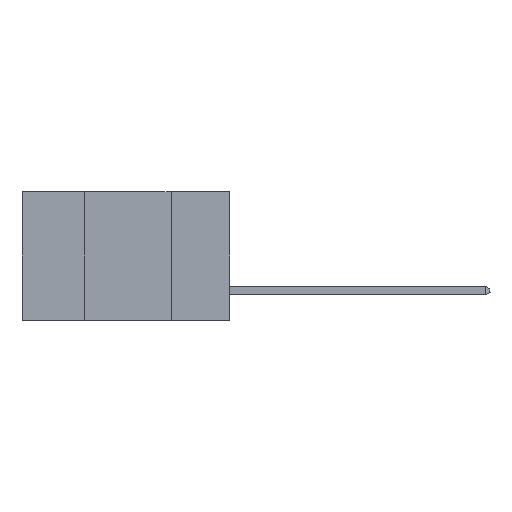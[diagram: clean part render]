
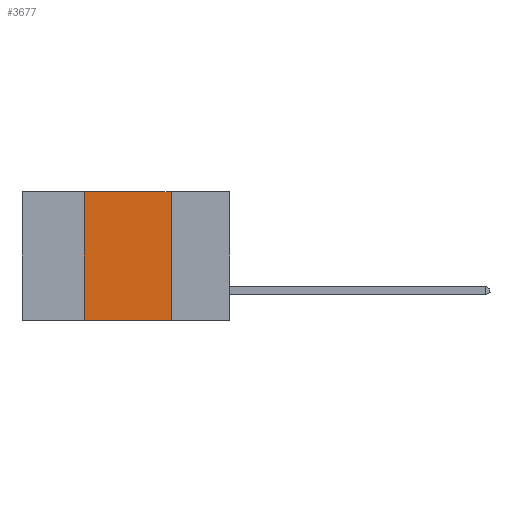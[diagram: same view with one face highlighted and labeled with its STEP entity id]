
A CAD part, left-side view. The second image highlights one B-rep face of the part: STEP entity #3677.
In plain terms, the highlighted planar face has unit normal (-1, 0, 0).
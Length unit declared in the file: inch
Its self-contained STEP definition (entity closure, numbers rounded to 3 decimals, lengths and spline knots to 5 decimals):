
#41 = VERTEX_POINT ( 'NONE', #5358 ) ;
#650 = LINE ( 'NONE', #7136, #1047 ) ;
#709 = LINE ( 'NONE', #8899, #6102 ) ;
#937 = LINE ( 'NONE', #3322, #4662 ) ;
#1047 = VECTOR ( 'NONE', #8446, 39.37008 ) ;
#1203 = AXIS2_PLACEMENT_3D ( 'NONE', #2027, #5406, #8885 ) ;
#2027 = CARTESIAN_POINT ( 'NONE',  ( 0., 0.6, 0. ) ) ;
#2568 = VECTOR ( 'NONE', #6865, 39.37008 ) ;
#2837 = ORIENTED_EDGE ( 'NONE', *, *, #5781, .F. ) ;
#2841 = LINE ( 'NONE', #6019, #2568 ) ;
#2975 = EDGE_CURVE ( 'NONE', #4807, #3349, #937, .T. ) ;
#3322 = CARTESIAN_POINT ( 'NONE',  ( 0., 0.17, 0. ) ) ;
#3349 = VERTEX_POINT ( 'NONE', #9101 ) ;
#3677 = ADVANCED_FACE ( 'NONE', ( #5063 ), #10851, .F. ) ;
#3805 = EDGE_CURVE ( 'NONE', #41, #3349, #650, .T. ) ;
#4180 = ORIENTED_EDGE ( 'NONE', *, *, #3805, .T. ) ;
#4305 = DIRECTION ( 'NONE',  ( 0., 0., -1. ) ) ;
#4662 = VECTOR ( 'NONE', #4305, 39.37008 ) ;
#4807 = VERTEX_POINT ( 'NONE', #8254 ) ;
#5063 = FACE_OUTER_BOUND ( 'NONE', #5847, .T. ) ;
#5358 = CARTESIAN_POINT ( 'NONE',  ( 0., 0.42, -0.37 ) ) ;
#5406 = DIRECTION ( 'NONE',  ( 1., 0., 0. ) ) ;
#5595 = VERTEX_POINT ( 'NONE', #6497 ) ;
#5781 = EDGE_CURVE ( 'NONE', #41, #5595, #2841, .T. ) ;
#5847 = EDGE_LOOP ( 'NONE', ( #8409, #8535, #2837, #4180 ) ) ;
#6019 = CARTESIAN_POINT ( 'NONE',  ( 0., 0.42, 0. ) ) ;
#6102 = VECTOR ( 'NONE', #9698, 39.37008 ) ;
#6497 = CARTESIAN_POINT ( 'NONE',  ( 0., 0.42, 0. ) ) ;
#6865 = DIRECTION ( 'NONE',  ( 0., 0., 1. ) ) ;
#7136 = CARTESIAN_POINT ( 'NONE',  ( 0., 0.6, -0.37 ) ) ;
#8254 = CARTESIAN_POINT ( 'NONE',  ( 0., 0.17, 0. ) ) ;
#8409 = ORIENTED_EDGE ( 'NONE', *, *, #2975, .F. ) ;
#8446 = DIRECTION ( 'NONE',  ( 0., -1., 0. ) ) ;
#8535 = ORIENTED_EDGE ( 'NONE', *, *, #9440, .F. ) ;
#8885 = DIRECTION ( 'NONE',  ( 0., 0., -1. ) ) ;
#8899 = CARTESIAN_POINT ( 'NONE',  ( 0., 0.6, 0. ) ) ;
#9101 = CARTESIAN_POINT ( 'NONE',  ( 0., 0.17, -0.37 ) ) ;
#9440 = EDGE_CURVE ( 'NONE', #5595, #4807, #709, .T. ) ;
#9698 = DIRECTION ( 'NONE',  ( 0., -1., 0. ) ) ;
#10851 = PLANE ( 'NONE',  #1203 ) ;
